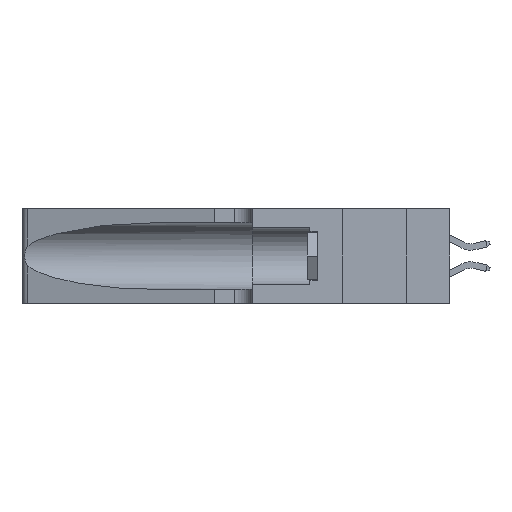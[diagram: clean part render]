
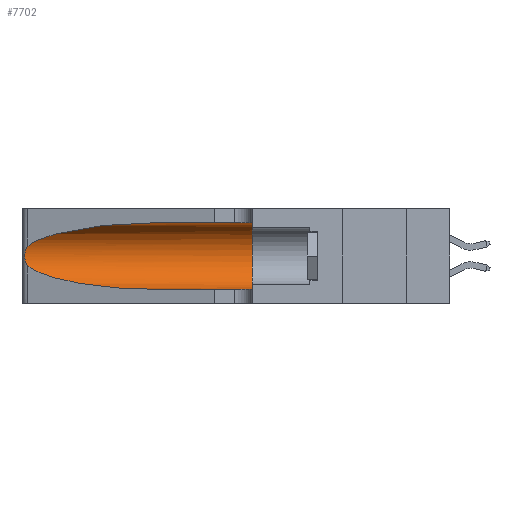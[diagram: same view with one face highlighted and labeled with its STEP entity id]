
A CAD part, left-side view. The second image highlights one B-rep face of the part: STEP entity #7702.
In plain terms, the highlighted cylindrical face has radius 3.308 mm (diameter 6.617 mm), a partial arc.
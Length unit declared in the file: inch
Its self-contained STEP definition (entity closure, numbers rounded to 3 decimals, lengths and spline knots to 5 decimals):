
#478 = CARTESIAN_POINT ( 'NONE',  ( 0.2373, 1.15595, 0.08982 ) ) ;
#726 = DIRECTION ( 'NONE',  ( 0., 0., -1. ) ) ;
#996 = CARTESIAN_POINT ( 'NONE',  ( 0.26075, 1.23896, 0.19203 ) ) ;
#1091 = CARTESIAN_POINT ( 'NONE',  ( 0.25789, 1.23486, 0.15765 ) ) ;
#1474 = EDGE_CURVE ( 'NONE', #5057, #18271, #12912, .T. ) ;
#1812 = CIRCLE ( 'NONE', #17273, 0.13025 ) ;
#2307 = EDGE_CURVE ( 'NONE', #17738, #18666, #1812, .T. ) ;
#2378 = DIRECTION ( 'NONE',  ( 0., 1., 0. ) ) ;
#2553 = CARTESIAN_POINT ( 'NONE',  ( 0.18966, 0.96281, 0.05475 ) ) ;
#2813 = DIRECTION ( 'NONE',  ( 0., -1., 0. ) ) ;
#3117 = CARTESIAN_POINT ( 'NONE',  ( 0.2373, 1.15595, 0.28018 ) ) ;
#3264 = CARTESIAN_POINT ( 'NONE',  ( 0.25639, 1.23186, 0.15144 ) ) ;
#4889 = LINE ( 'NONE', #22772, #13853 ) ;
#4911 = EDGE_LOOP ( 'NONE', ( #11306, #5958, #15994, #7582, #23609, #12400 ) ) ;
#5057 = VERTEX_POINT ( 'NONE', #10694 ) ;
#5362 = VERTEX_POINT ( 'NONE', #5516 ) ;
#5516 = CARTESIAN_POINT ( 'NONE',  ( 0.1305, 0.72297, 0.31525 ) ) ;
#5958 = ORIENTED_EDGE ( 'NONE', *, *, #1474, .T. ) ;
#6988 = CARTESIAN_POINT ( 'NONE',  ( 0.1305, 0.72297, 0.05475 ) ) ;
#7176 = CARTESIAN_POINT ( 'NONE',  ( 0.26018, 1.23835, 0.19895 ) ) ;
#7212 = VERTEX_POINT ( 'NONE', #6988 ) ;
#7270 = CARTESIAN_POINT ( 'NONE',  ( 0.25639, 1.23184, 0.21858 ) ) ;
#7582 = ORIENTED_EDGE ( 'NONE', *, *, #10338, .T. ) ;
#7702 = ADVANCED_FACE ( 'NONE', ( #8653 ), #12801, .F. ) ;
#7748 = EDGE_CURVE ( 'NONE', #5362, #17738, #14425, .T. ) ;
#8376 = CARTESIAN_POINT ( 'NONE',  ( 0.1305, 0.72297, 0.05475 ) ) ;
#8450 =( BOUNDED_CURVE ( )  B_SPLINE_CURVE ( 3, ( #23522, #15338, #3117, #25530 ),
 .UNSPECIFIED., .F., .T. ) 
 B_SPLINE_CURVE_WITH_KNOTS ( ( 4, 4 ),
 ( 1.5708, 2.84003 ),
 .UNSPECIFIED. ) 
 CURVE ( )  GEOMETRIC_REPRESENTATION_ITEM ( )  RATIONAL_B_SPLINE_CURVE ( ( 1., 0.87, 0.87, 1. ) ) 
 REPRESENTATION_ITEM ( '' )  );
#8653 = FACE_OUTER_BOUND ( 'NONE', #4911, .T. ) ;
#10027 = EDGE_CURVE ( 'NONE', #5362, #5057, #8450, .T. ) ;
#10338 = EDGE_CURVE ( 'NONE', #7212, #18666, #4889, .T. ) ;
#10558 = CARTESIAN_POINT ( 'NONE',  ( 0.1305, 0.35, 0.05475 ) ) ;
#10694 = CARTESIAN_POINT ( 'NONE',  ( 0.25487, 1.22718, 0.22369 ) ) ;
#11123 = CARTESIAN_POINT ( 'NONE',  ( 0.26075, 1.23896, 0.178 ) ) ;
#11306 = ORIENTED_EDGE ( 'NONE', *, *, #10027, .T. ) ;
#12272 = CARTESIAN_POINT ( 'NONE',  ( 0.25487, 1.22718, 0.14631 ) ) ;
#12400 = ORIENTED_EDGE ( 'NONE', *, *, #7748, .F. ) ;
#12801 = CYLINDRICAL_SURFACE ( 'NONE', #13777, 0.13025 ) ;
#12912 = B_SPLINE_CURVE_WITH_KNOTS ( 'NONE', 3,
 ( #21651, #15490, #7270, #19249, #23675, #7176, #996, #11123, #21553, #25322, #1091, #3264, #19614, #23494 ),
 .UNSPECIFIED., .F., .F.,
 ( 4, 2, 2, 2, 2, 2, 4 ),
 ( 0., 0.00027, 0.00053, 0.00107, 0.0016, 0.00187, 0.00214 ),
 .UNSPECIFIED. ) ;
#13777 = AXIS2_PLACEMENT_3D ( 'NONE', #18971, #2813, #726 ) ;
#13853 = VECTOR ( 'NONE', #20487, 39.37008 ) ;
#14201 = CARTESIAN_POINT ( 'NONE',  ( 0.1305, 0.35, 0.185 ) ) ;
#14425 = LINE ( 'NONE', #14952, #20522 ) ;
#14952 = CARTESIAN_POINT ( 'NONE',  ( 0.1305, 1.61858, 0.31525 ) ) ;
#15228 = DIRECTION ( 'NONE',  ( 0., -1., 0. ) ) ;
#15338 = CARTESIAN_POINT ( 'NONE',  ( 0.18966, 0.96281, 0.31525 ) ) ;
#15490 = CARTESIAN_POINT ( 'NONE',  ( 0.25555, 1.22994, 0.2215 ) ) ;
#15616 = EDGE_CURVE ( 'NONE', #18271, #7212, #18754, .T. ) ;
#15994 = ORIENTED_EDGE ( 'NONE', *, *, #15616, .T. ) ;
#16763 = DIRECTION ( 'NONE',  ( 0., 0., 1. ) ) ;
#17273 = AXIS2_PLACEMENT_3D ( 'NONE', #14201, #2378, #16763 ) ;
#17738 = VERTEX_POINT ( 'NONE', #22643 ) ;
#18271 = VERTEX_POINT ( 'NONE', #12272 ) ;
#18666 = VERTEX_POINT ( 'NONE', #10558 ) ;
#18754 =( BOUNDED_CURVE ( )  B_SPLINE_CURVE ( 3, ( #24668, #478, #2553, #8376 ),
 .UNSPECIFIED., .F., .F. ) 
 B_SPLINE_CURVE_WITH_KNOTS ( ( 4, 4 ),
 ( 3.44316, 4.71239 ),
 .UNSPECIFIED. ) 
 CURVE ( )  GEOMETRIC_REPRESENTATION_ITEM ( )  RATIONAL_B_SPLINE_CURVE ( ( 1., 0.87, 0.87, 1. ) ) 
 REPRESENTATION_ITEM ( '' )  );
#18971 = CARTESIAN_POINT ( 'NONE',  ( 0.1305, 1.61858, 0.185 ) ) ;
#19249 = CARTESIAN_POINT ( 'NONE',  ( 0.25787, 1.23484, 0.2124 ) ) ;
#19614 = CARTESIAN_POINT ( 'NONE',  ( 0.25555, 1.22993, 0.14849 ) ) ;
#20487 = DIRECTION ( 'NONE',  ( 0., -1., 0. ) ) ;
#20522 = VECTOR ( 'NONE', #15228, 39.37008 ) ;
#21553 = CARTESIAN_POINT ( 'NONE',  ( 0.26017, 1.23833, 0.17102 ) ) ;
#21651 = CARTESIAN_POINT ( 'NONE',  ( 0.25487, 1.22718, 0.22369 ) ) ;
#22643 = CARTESIAN_POINT ( 'NONE',  ( 0.1305, 0.35, 0.31525 ) ) ;
#22772 = CARTESIAN_POINT ( 'NONE',  ( 0.1305, 1.61858, 0.05475 ) ) ;
#23494 = CARTESIAN_POINT ( 'NONE',  ( 0.25487, 1.22718, 0.14631 ) ) ;
#23522 = CARTESIAN_POINT ( 'NONE',  ( 0.1305, 0.72297, 0.31525 ) ) ;
#23609 = ORIENTED_EDGE ( 'NONE', *, *, #2307, .F. ) ;
#23675 = CARTESIAN_POINT ( 'NONE',  ( 0.25854, 1.2359, 0.20912 ) ) ;
#24668 = CARTESIAN_POINT ( 'NONE',  ( 0.25487, 1.22718, 0.14631 ) ) ;
#25322 = CARTESIAN_POINT ( 'NONE',  ( 0.25856, 1.23593, 0.16098 ) ) ;
#25530 = CARTESIAN_POINT ( 'NONE',  ( 0.25487, 1.22718, 0.22369 ) ) ;
